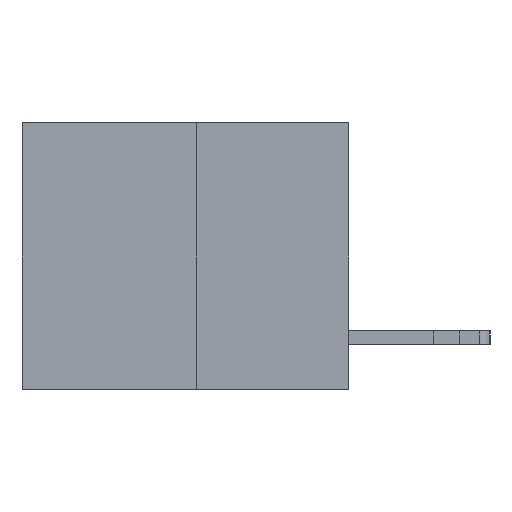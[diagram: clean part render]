
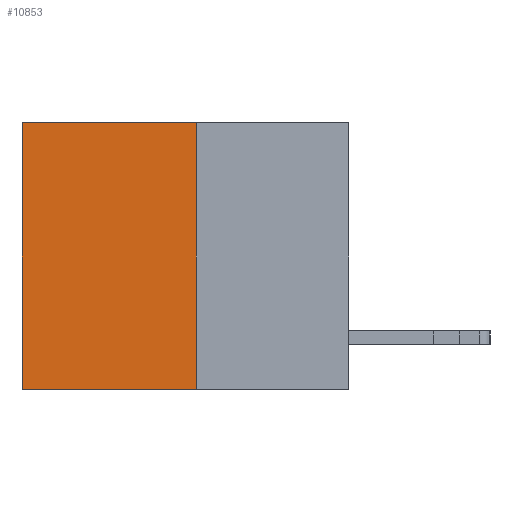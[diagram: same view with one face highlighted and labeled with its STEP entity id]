
A CAD part, left-side view. The second image highlights one B-rep face of the part: STEP entity #10853.
In plain terms, the highlighted planar face has unit normal (-1, 0, 0).
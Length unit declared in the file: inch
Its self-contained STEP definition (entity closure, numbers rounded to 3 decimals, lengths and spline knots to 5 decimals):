
#76 = AXIS2_PLACEMENT_3D ( 'NONE', #10072, #8091, #357 ) ;
#168 = CARTESIAN_POINT ( 'NONE',  ( 0.3165, 0.28, 0. ) ) ;
#357 = DIRECTION ( 'NONE',  ( 0., 0., -1. ) ) ;
#1192 = DIRECTION ( 'NONE',  ( 0., 1., 0. ) ) ;
#2070 = EDGE_CURVE ( 'NONE', #16495, #23949, #14049, .T. ) ;
#3646 = LINE ( 'NONE', #168, #21014 ) ;
#4675 = ORIENTED_EDGE ( 'NONE', *, *, #5218, .F. ) ;
#5218 = EDGE_CURVE ( 'NONE', #23949, #22200, #7417, .T. ) ;
#6100 = PLANE ( 'NONE',  #76 ) ;
#7249 = VERTEX_POINT ( 'NONE', #24880 ) ;
#7417 = LINE ( 'NONE', #13067, #18243 ) ;
#7923 = VECTOR ( 'NONE', #10308, 39.37008 ) ;
#8091 = DIRECTION ( 'NONE',  ( 1., 0., 0. ) ) ;
#8337 = CARTESIAN_POINT ( 'NONE',  ( 0.3165, 0.6, -0.49 ) ) ;
#10072 = CARTESIAN_POINT ( 'NONE',  ( 0.3165, 0.28, -0.49 ) ) ;
#10308 = DIRECTION ( 'NONE',  ( 0., 0., -1. ) ) ;
#10853 = ADVANCED_FACE ( 'NONE', ( #20360 ), #6100, .F. ) ;
#11643 = EDGE_CURVE ( 'NONE', #7249, #22200, #13186, .T. ) ;
#13067 = CARTESIAN_POINT ( 'NONE',  ( 0.3165, 0.28, -0.49 ) ) ;
#13186 = LINE ( 'NONE', #8337, #7923 ) ;
#14049 = LINE ( 'NONE', #22561, #19933 ) ;
#14892 = ORIENTED_EDGE ( 'NONE', *, *, #2070, .F. ) ;
#15062 = CARTESIAN_POINT ( 'NONE',  ( 0.3165, 0.6, -0.49 ) ) ;
#15720 = ORIENTED_EDGE ( 'NONE', *, *, #20516, .T. ) ;
#15804 = CARTESIAN_POINT ( 'NONE',  ( 0.3165, 0.28, -0.49 ) ) ;
#16495 = VERTEX_POINT ( 'NONE', #24588 ) ;
#17938 = DIRECTION ( 'NONE',  ( 0., 1., 0. ) ) ;
#18104 = ORIENTED_EDGE ( 'NONE', *, *, #11643, .T. ) ;
#18243 = VECTOR ( 'NONE', #1192, 39.37008 ) ;
#19933 = VECTOR ( 'NONE', #21519, 39.37008 ) ;
#20360 = FACE_OUTER_BOUND ( 'NONE', #22736, .T. ) ;
#20516 = EDGE_CURVE ( 'NONE', #16495, #7249, #3646, .T. ) ;
#21014 = VECTOR ( 'NONE', #17938, 39.37008 ) ;
#21519 = DIRECTION ( 'NONE',  ( 0., 0., -1. ) ) ;
#22200 = VERTEX_POINT ( 'NONE', #15062 ) ;
#22561 = CARTESIAN_POINT ( 'NONE',  ( 0.3165, 0.28, -0.49 ) ) ;
#22736 = EDGE_LOOP ( 'NONE', ( #18104, #4675, #14892, #15720 ) ) ;
#23949 = VERTEX_POINT ( 'NONE', #15804 ) ;
#24588 = CARTESIAN_POINT ( 'NONE',  ( 0.3165, 0.28, 0. ) ) ;
#24880 = CARTESIAN_POINT ( 'NONE',  ( 0.3165, 0.6, 0. ) ) ;
